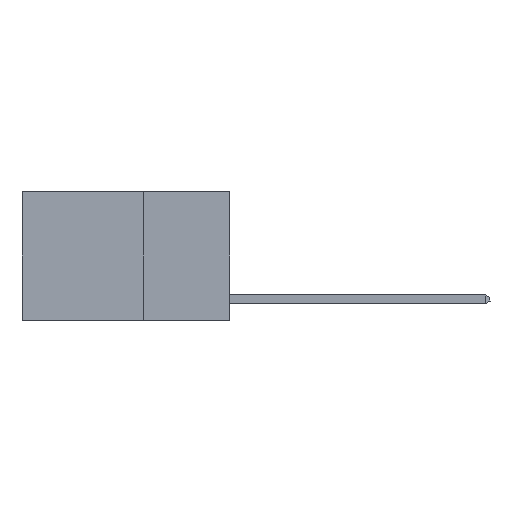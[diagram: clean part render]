
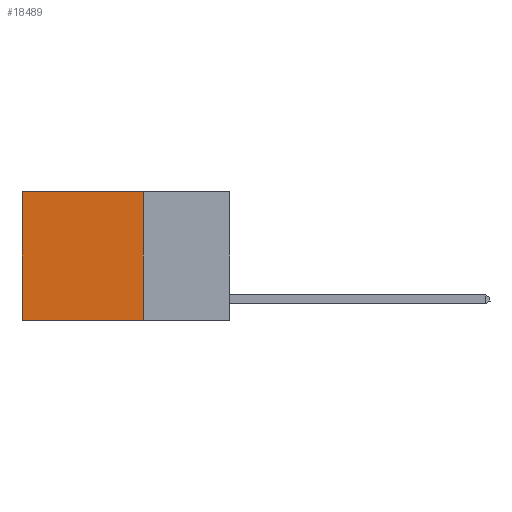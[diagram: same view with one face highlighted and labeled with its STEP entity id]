
A CAD part, left-side view. The second image highlights one B-rep face of the part: STEP entity #18489.
In plain terms, the highlighted planar face has unit normal (-1, 0, 0).
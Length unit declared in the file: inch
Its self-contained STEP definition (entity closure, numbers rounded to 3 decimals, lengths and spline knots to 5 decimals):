
#120 = EDGE_CURVE ( 'NONE', #12720, #24765, #16631, .T. ) ;
#355 = CARTESIAN_POINT ( 'NONE',  ( 0.2625, 0.25, 0. ) ) ;
#401 = LINE ( 'NONE', #6578, #13655 ) ;
#1759 = VERTEX_POINT ( 'NONE', #23721 ) ;
#2040 = EDGE_CURVE ( 'NONE', #1759, #17933, #401, .T. ) ;
#2426 = CARTESIAN_POINT ( 'NONE',  ( 0.2625, 0.6, 0. ) ) ;
#3144 = DIRECTION ( 'NONE',  ( 0., 0., -1. ) ) ;
#5916 = VECTOR ( 'NONE', #21568, 39.37008 ) ;
#6578 = CARTESIAN_POINT ( 'NONE',  ( 0.2625, 0.25, -0.37 ) ) ;
#6715 = CARTESIAN_POINT ( 'NONE',  ( 0.2625, 0.25, 0. ) ) ;
#7147 = CARTESIAN_POINT ( 'NONE',  ( 0.2625, 0.25, 0. ) ) ;
#8656 = LINE ( 'NONE', #355, #15161 ) ;
#8911 = EDGE_CURVE ( 'NONE', #24765, #17933, #25609, .T. ) ;
#9064 = CARTESIAN_POINT ( 'NONE',  ( 0.2625, 0.6, -0.37 ) ) ;
#9160 = PLANE ( 'NONE',  #14025 ) ;
#9685 = EDGE_CURVE ( 'NONE', #12720, #1759, #8656, .T. ) ;
#10782 = DIRECTION ( 'NONE',  ( 1., 0., 0. ) ) ;
#12066 = ORIENTED_EDGE ( 'NONE', *, *, #9685, .F. ) ;
#12720 = VERTEX_POINT ( 'NONE', #22135 ) ;
#13655 = VECTOR ( 'NONE', #24942, 39.37008 ) ;
#14025 = AXIS2_PLACEMENT_3D ( 'NONE', #7147, #10782, #3144 ) ;
#14970 = ORIENTED_EDGE ( 'NONE', *, *, #8911, .T. ) ;
#15161 = VECTOR ( 'NONE', #25029, 39.37008 ) ;
#15545 = CARTESIAN_POINT ( 'NONE',  ( 0.2625, 0.6, 0. ) ) ;
#16631 = LINE ( 'NONE', #6715, #22667 ) ;
#17068 = FACE_OUTER_BOUND ( 'NONE', #24389, .T. ) ;
#17933 = VERTEX_POINT ( 'NONE', #9064 ) ;
#18489 = ADVANCED_FACE ( 'NONE', ( #17068 ), #9160, .F. ) ;
#21568 = DIRECTION ( 'NONE',  ( 0., 0., -1. ) ) ;
#22135 = CARTESIAN_POINT ( 'NONE',  ( 0.2625, 0.25, 0. ) ) ;
#22667 = VECTOR ( 'NONE', #25079, 39.37008 ) ;
#23721 = CARTESIAN_POINT ( 'NONE',  ( 0.2625, 0.25, -0.37 ) ) ;
#24389 = EDGE_LOOP ( 'NONE', ( #14970, #26383, #12066, #25984 ) ) ;
#24765 = VERTEX_POINT ( 'NONE', #2426 ) ;
#24942 = DIRECTION ( 'NONE',  ( 0., 1., 0. ) ) ;
#25029 = DIRECTION ( 'NONE',  ( 0., 0., -1. ) ) ;
#25079 = DIRECTION ( 'NONE',  ( 0., 1., 0. ) ) ;
#25609 = LINE ( 'NONE', #15545, #5916 ) ;
#25984 = ORIENTED_EDGE ( 'NONE', *, *, #120, .T. ) ;
#26383 = ORIENTED_EDGE ( 'NONE', *, *, #2040, .F. ) ;
